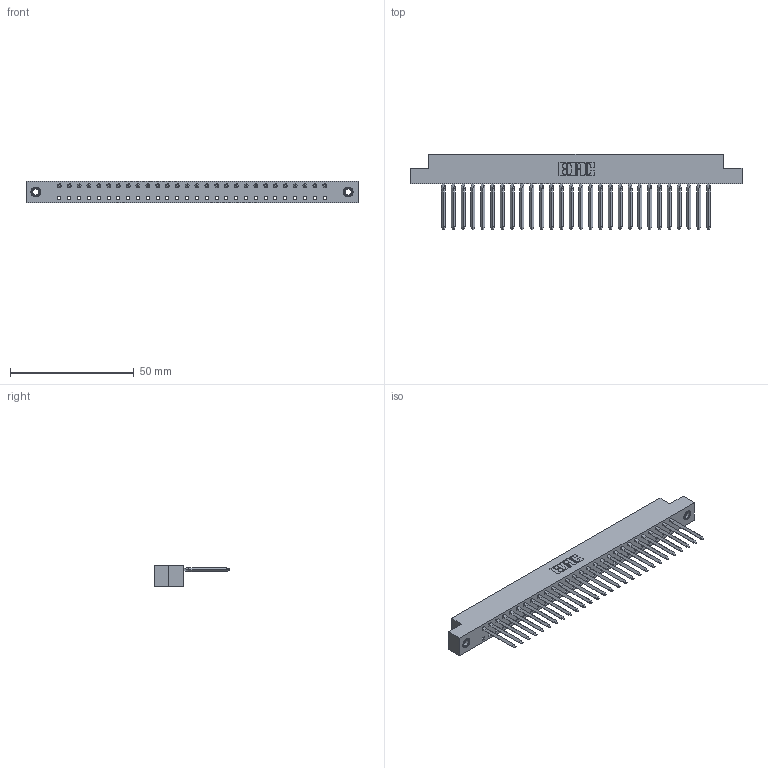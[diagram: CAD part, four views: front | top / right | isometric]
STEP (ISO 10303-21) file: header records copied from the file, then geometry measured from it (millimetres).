
FILE_DESCRIPTION (( 'STEP AP203' ), '1' );
FILE_NAME ('338-028-541-107.STEP', '2020-03-24T18:00:35', ( '' ), ( '' ), 'SwSTEP 2.0', 'SolidWorks 2016', '' );
FILE_SCHEMA (( 'CONFIG_CONTROL_DESIGN' ));
Length unit declared in the file: inch
Products named in the file (4): 338-028-541-107; 345-250-001_345-250-005-103; 338-210-001_338-210-028-004; 338-290-001_541
Assembly tree (31 placements, depth 2):
  338-028-541-107
    338-210-001_338-210-028-004
    338-290-001_541  x28
    345-250-001_345-250-005-103  x2
Bounding box: 133.96 x 30.56 x 8.71 mm (x, y, z)
Volume: 9386.9 mm3; surface area: 15414.6 mm2
Topology: 31 solids, 31 shells, 2758 faces, 7583 edges, 4842 vertices
Faces by surface type: plane 1902, cylinder 728, bspline 112, cone 12, torus 4
Entity records: 56297 total; most frequent: CARTESIAN_POINT 11255, ORIENTED_EDGE 9504, DIRECTION 8885, EDGE_CURVE 4752, VECTOR 3553, LINE 3553, VERTEX_POINT 3084, AXIS2_PLACEMENT_3D 2666
